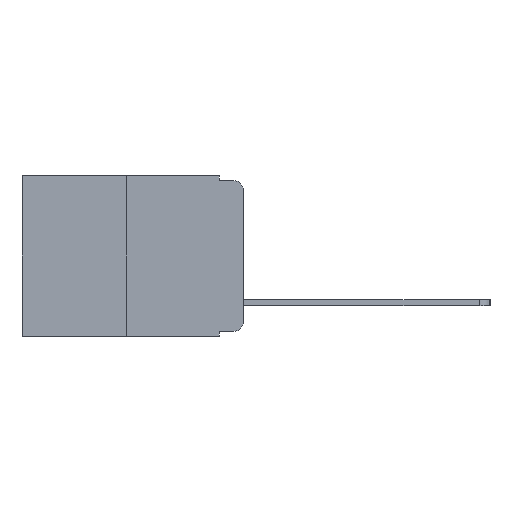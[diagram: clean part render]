
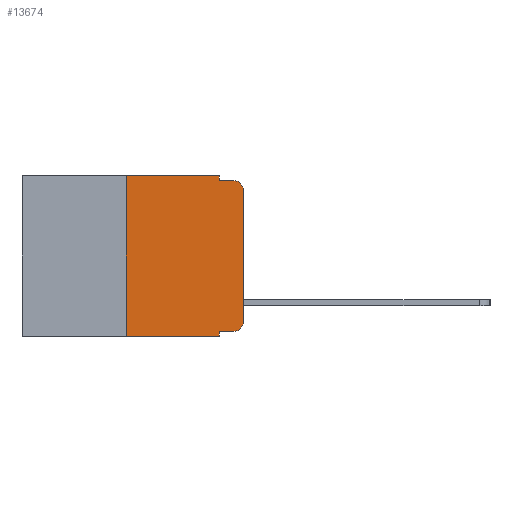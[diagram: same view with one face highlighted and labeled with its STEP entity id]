
A CAD part, left-side view. The second image highlights one B-rep face of the part: STEP entity #13674.
In plain terms, the highlighted planar face has unit normal (-1, 0, 0).
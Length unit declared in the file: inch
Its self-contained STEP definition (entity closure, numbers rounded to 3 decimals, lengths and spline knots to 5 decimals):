
#84 = VECTOR ( 'NONE', #15623, 39.37008 ) ;
#322 = ORIENTED_EDGE ( 'NONE', *, *, #10972, .F. ) ;
#439 = DIRECTION ( 'NONE',  ( 0., 0., -1. ) ) ;
#495 = VERTEX_POINT ( 'NONE', #6045 ) ;
#627 = CARTESIAN_POINT ( 'NONE',  ( 0., 0.051, -0.333 ) ) ;
#823 = ORIENTED_EDGE ( 'NONE', *, *, #11067, .F. ) ;
#1111 = DIRECTION ( 'NONE',  ( 0., -1., 0. ) ) ;
#1755 = ORIENTED_EDGE ( 'NONE', *, *, #8659, .T. ) ;
#1963 = CARTESIAN_POINT ( 'NONE',  ( 0., 0.473, 0. ) ) ;
#2103 = DIRECTION ( 'NONE',  ( 0., -1., 0. ) ) ;
#2414 = CARTESIAN_POINT ( 'NONE',  ( 0., 0.02, -0.313 ) ) ;
#2475 = VECTOR ( 'NONE', #2103, 39.37008 ) ;
#2690 = CARTESIAN_POINT ( 'NONE',  ( 0., 0.25, -0.343 ) ) ;
#3099 = DIRECTION ( 'NONE',  ( 0., -1., 0. ) ) ;
#3357 = PLANE ( 'NONE',  #12863 ) ;
#3629 = VERTEX_POINT ( 'NONE', #7590 ) ;
#3747 = DIRECTION ( 'NONE',  ( 0., 0., -1. ) ) ;
#4071 = CARTESIAN_POINT ( 'NONE',  ( 0., 0.25, 0. ) ) ;
#4102 = VERTEX_POINT ( 'NONE', #627 ) ;
#4473 = ORIENTED_EDGE ( 'NONE', *, *, #15544, .T. ) ;
#4625 = DIRECTION ( 'NONE',  ( 0., 0., -1. ) ) ;
#4881 = ORIENTED_EDGE ( 'NONE', *, *, #10265, .F. ) ;
#5488 = VERTEX_POINT ( 'NONE', #11436 ) ;
#5865 = CARTESIAN_POINT ( 'NONE',  ( 0., 0.25, 0. ) ) ;
#5902 = DIRECTION ( 'NONE',  ( 1., 0., 0. ) ) ;
#6045 = CARTESIAN_POINT ( 'NONE',  ( 0., 0., -0.03 ) ) ;
#6096 = VECTOR ( 'NONE', #3099, 39.37008 ) ;
#6738 = ORIENTED_EDGE ( 'NONE', *, *, #13458, .T. ) ;
#6778 = DIRECTION ( 'NONE',  ( -1., 0., 0. ) ) ;
#7148 = ORIENTED_EDGE ( 'NONE', *, *, #12680, .F. ) ;
#7183 = DIRECTION ( 'NONE',  ( 0., 0., 1. ) ) ;
#7333 = LINE ( 'NONE', #14433, #84 ) ;
#7448 = AXIS2_PLACEMENT_3D ( 'NONE', #14057, #6778, #15253 ) ;
#7590 = CARTESIAN_POINT ( 'NONE',  ( 0., 0.02, -0.333 ) ) ;
#8191 = VECTOR ( 'NONE', #13035, 39.37008 ) ;
#8201 = CARTESIAN_POINT ( 'NONE',  ( 0., 0.02, -0.01 ) ) ;
#8248 = DIRECTION ( 'NONE',  ( 0., 0., 1. ) ) ;
#8659 = EDGE_CURVE ( 'NONE', #3629, #11202, #11963, .T. ) ;
#8723 = VECTOR ( 'NONE', #7183, 39.37008 ) ;
#9013 = AXIS2_PLACEMENT_3D ( 'NONE', #2414, #11284, #3747 ) ;
#9068 = CIRCLE ( 'NONE', #7448, 0.02 ) ;
#9276 = VECTOR ( 'NONE', #439, 39.37008 ) ;
#9318 = VERTEX_POINT ( 'NONE', #10815 ) ;
#9464 = EDGE_CURVE ( 'NONE', #4102, #3629, #12885, .T. ) ;
#9470 = LINE ( 'NONE', #13094, #6096 ) ;
#9601 = FACE_OUTER_BOUND ( 'NONE', #11331, .T. ) ;
#9666 = ORIENTED_EDGE ( 'NONE', *, *, #14258, .T. ) ;
#9818 = CARTESIAN_POINT ( 'NONE',  ( 0., 0.051, -0.333 ) ) ;
#10095 = VERTEX_POINT ( 'NONE', #8201 ) ;
#10265 = EDGE_CURVE ( 'NONE', #4102, #9318, #7333, .T. ) ;
#10815 = CARTESIAN_POINT ( 'NONE',  ( 0., 0.051, -0.343 ) ) ;
#10918 = LINE ( 'NONE', #16126, #12615 ) ;
#10972 = EDGE_CURVE ( 'NONE', #14054, #5488, #9470, .T. ) ;
#11067 = EDGE_CURVE ( 'NONE', #11539, #14054, #14688, .T. ) ;
#11202 = VERTEX_POINT ( 'NONE', #15757 ) ;
#11280 = VECTOR ( 'NONE', #8248, 39.37008 ) ;
#11284 = DIRECTION ( 'NONE',  ( -1., 0., 0. ) ) ;
#11331 = EDGE_LOOP ( 'NONE', ( #9666, #6738, #7148, #13601, #322, #823, #4473, #4881, #14715, #1755 ) ) ;
#11436 = CARTESIAN_POINT ( 'NONE',  ( 0., 0.051, 0. ) ) ;
#11539 = VERTEX_POINT ( 'NONE', #2690 ) ;
#11830 = CARTESIAN_POINT ( 'NONE',  ( 0., 0.473, -0.343 ) ) ;
#11879 = EDGE_CURVE ( 'NONE', #5488, #16212, #15579, .T. ) ;
#11909 = CARTESIAN_POINT ( 'NONE',  ( 0., 0., 0. ) ) ;
#11963 = CIRCLE ( 'NONE', #9013, 0.02 ) ;
#12615 = VECTOR ( 'NONE', #1111, 39.37008 ) ;
#12650 = CARTESIAN_POINT ( 'NONE',  ( 0., 0.051, -0.01 ) ) ;
#12680 = EDGE_CURVE ( 'NONE', #16212, #10095, #10918, .T. ) ;
#12863 = AXIS2_PLACEMENT_3D ( 'NONE', #1963, #5902, #4625 ) ;
#12885 = LINE ( 'NONE', #9818, #2475 ) ;
#13035 = DIRECTION ( 'NONE',  ( 0., -1., 0. ) ) ;
#13094 = CARTESIAN_POINT ( 'NONE',  ( 0., 0.473, 0. ) ) ;
#13270 = CARTESIAN_POINT ( 'NONE',  ( 0., 0.051, 0. ) ) ;
#13458 = EDGE_CURVE ( 'NONE', #495, #10095, #9068, .T. ) ;
#13601 = ORIENTED_EDGE ( 'NONE', *, *, #11879, .F. ) ;
#13674 = ADVANCED_FACE ( 'NONE', ( #9601 ), #3357, .F. ) ;
#14054 = VERTEX_POINT ( 'NONE', #4071 ) ;
#14057 = CARTESIAN_POINT ( 'NONE',  ( 0., 0.02, -0.03 ) ) ;
#14258 = EDGE_CURVE ( 'NONE', #11202, #495, #14423, .T. ) ;
#14423 = LINE ( 'NONE', #11909, #11280 ) ;
#14433 = CARTESIAN_POINT ( 'NONE',  ( 0., 0.051, 0. ) ) ;
#14570 = LINE ( 'NONE', #11830, #8191 ) ;
#14688 = LINE ( 'NONE', #5865, #8723 ) ;
#14715 = ORIENTED_EDGE ( 'NONE', *, *, #9464, .T. ) ;
#15253 = DIRECTION ( 'NONE',  ( 0., 0., -1. ) ) ;
#15544 = EDGE_CURVE ( 'NONE', #11539, #9318, #14570, .T. ) ;
#15579 = LINE ( 'NONE', #13270, #9276 ) ;
#15623 = DIRECTION ( 'NONE',  ( 0., 0., -1. ) ) ;
#15757 = CARTESIAN_POINT ( 'NONE',  ( 0., 0., -0.313 ) ) ;
#16126 = CARTESIAN_POINT ( 'NONE',  ( 0., 0.051, -0.01 ) ) ;
#16212 = VERTEX_POINT ( 'NONE', #12650 ) ;
